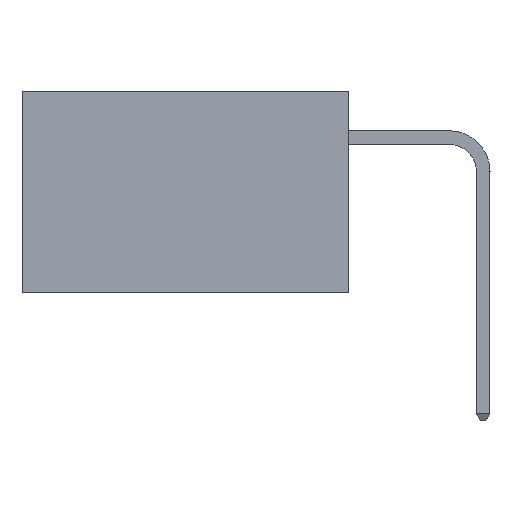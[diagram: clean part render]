
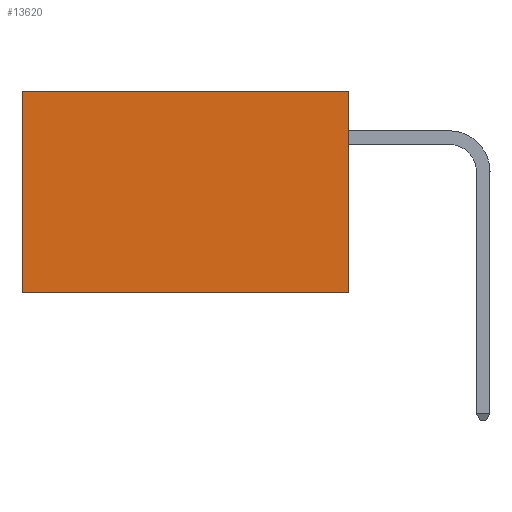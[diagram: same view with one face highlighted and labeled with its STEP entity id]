
A CAD part, left-side view. The second image highlights one B-rep face of the part: STEP entity #13620.
In plain terms, the highlighted planar face has unit normal (-1, 0, 0).
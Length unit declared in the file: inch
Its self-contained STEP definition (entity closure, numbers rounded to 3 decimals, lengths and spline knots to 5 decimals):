
#240 = ORIENTED_EDGE ( 'NONE', *, *, #9803, .T. ) ;
#321 = PLANE ( 'NONE',  #18018 ) ;
#750 = LINE ( 'NONE', #17732, #14452 ) ;
#895 = CARTESIAN_POINT ( 'NONE',  ( 0.2875, 0., -0.37 ) ) ;
#1497 = CARTESIAN_POINT ( 'NONE',  ( 0.2875, 0., 0. ) ) ;
#1576 = EDGE_CURVE ( 'NONE', #11020, #11465, #14572, .T. ) ;
#1883 = DIRECTION ( 'NONE',  ( 0., 0., -1. ) ) ;
#1997 = VECTOR ( 'NONE', #2835, 39.37008 ) ;
#2835 = DIRECTION ( 'NONE',  ( 0., 0., -1. ) ) ;
#3013 = ORIENTED_EDGE ( 'NONE', *, *, #1576, .F. ) ;
#3672 = LINE ( 'NONE', #18699, #13983 ) ;
#4364 = CARTESIAN_POINT ( 'NONE',  ( 0.2875, 0.6, 0. ) ) ;
#4715 = EDGE_CURVE ( 'NONE', #19566, #20097, #750, .T. ) ;
#5958 = CARTESIAN_POINT ( 'NONE',  ( 0.2875, 0.6, -0.37 ) ) ;
#6128 = FACE_OUTER_BOUND ( 'NONE', #14234, .T. ) ;
#8601 = DIRECTION ( 'NONE',  ( 0., 1., 0. ) ) ;
#8663 = CARTESIAN_POINT ( 'NONE',  ( 0.2875, 0., -0.37 ) ) ;
#8822 = LINE ( 'NONE', #12303, #1997 ) ;
#9803 = EDGE_CURVE ( 'NONE', #20097, #11465, #8822, .T. ) ;
#9807 = EDGE_CURVE ( 'NONE', #19566, #11020, #3672, .T. ) ;
#11020 = VERTEX_POINT ( 'NONE', #895 ) ;
#11465 = VERTEX_POINT ( 'NONE', #5958 ) ;
#12303 = CARTESIAN_POINT ( 'NONE',  ( 0.2875, 0.6, 0. ) ) ;
#13059 = CARTESIAN_POINT ( 'NONE',  ( 0.2875, 0., 0. ) ) ;
#13352 = VECTOR ( 'NONE', #8601, 39.37008 ) ;
#13505 = ORIENTED_EDGE ( 'NONE', *, *, #4715, .T. ) ;
#13620 = ADVANCED_FACE ( 'NONE', ( #6128 ), #321, .F. ) ;
#13983 = VECTOR ( 'NONE', #14445, 39.37008 ) ;
#14234 = EDGE_LOOP ( 'NONE', ( #240, #3013, #19920, #13505 ) ) ;
#14335 = DIRECTION ( 'NONE',  ( 1., 0., 0. ) ) ;
#14445 = DIRECTION ( 'NONE',  ( 0., 0., -1. ) ) ;
#14452 = VECTOR ( 'NONE', #18119, 39.37008 ) ;
#14572 = LINE ( 'NONE', #8663, #13352 ) ;
#17732 = CARTESIAN_POINT ( 'NONE',  ( 0.2875, 0., 0. ) ) ;
#18018 = AXIS2_PLACEMENT_3D ( 'NONE', #13059, #14335, #1883 ) ;
#18119 = DIRECTION ( 'NONE',  ( 0., 1., 0. ) ) ;
#18699 = CARTESIAN_POINT ( 'NONE',  ( 0.2875, 0., 0. ) ) ;
#19566 = VERTEX_POINT ( 'NONE', #1497 ) ;
#19920 = ORIENTED_EDGE ( 'NONE', *, *, #9807, .F. ) ;
#20097 = VERTEX_POINT ( 'NONE', #4364 ) ;
